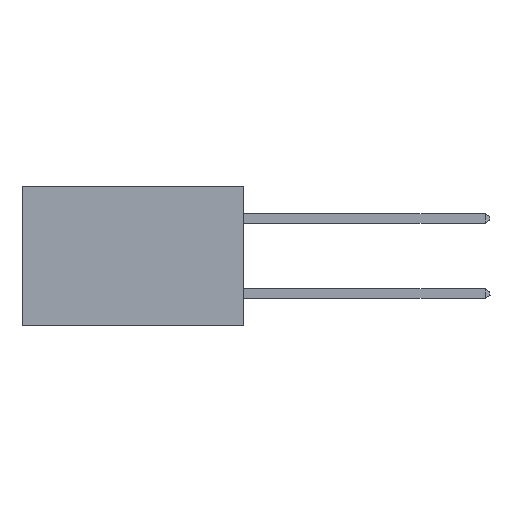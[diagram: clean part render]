
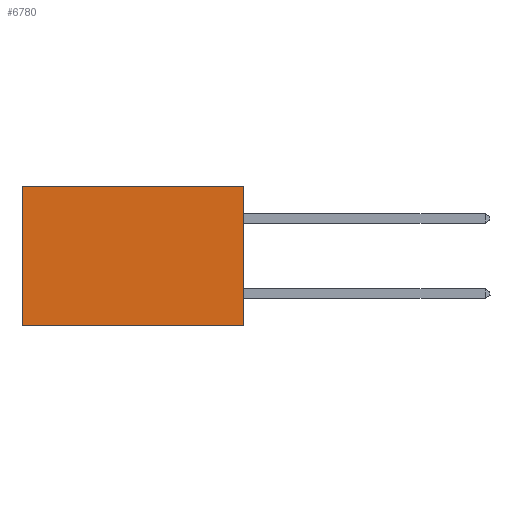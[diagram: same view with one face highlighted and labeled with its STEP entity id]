
A CAD part, left-side view. The second image highlights one B-rep face of the part: STEP entity #6780.
In plain terms, the highlighted planar face has unit normal (-1, 0, 0).
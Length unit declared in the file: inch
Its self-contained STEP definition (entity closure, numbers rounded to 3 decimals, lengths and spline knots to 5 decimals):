
#220 = AXIS2_PLACEMENT_3D ( 'NONE', #2139, #3180, #7868 ) ;
#2125 = CARTESIAN_POINT ( 'NONE',  ( 0.277, 0.59, -0.37 ) ) ;
#2139 = CARTESIAN_POINT ( 'NONE',  ( 0.277, 0., -0.37 ) ) ;
#2265 = FACE_OUTER_BOUND ( 'NONE', #10763, .T. ) ;
#2348 = LINE ( 'NONE', #7175, #12585 ) ;
#2513 = DIRECTION ( 'NONE',  ( 0., 0., -1. ) ) ;
#3180 = DIRECTION ( 'NONE',  ( 1., 0., 0. ) ) ;
#3348 = DIRECTION ( 'NONE',  ( 0., 1., 0. ) ) ;
#4469 = PLANE ( 'NONE',  #220 ) ;
#5017 = VERTEX_POINT ( 'NONE', #2125 ) ;
#6780 = ADVANCED_FACE ( 'NONE', ( #2265 ), #4469, .F. ) ;
#7138 = CARTESIAN_POINT ( 'NONE',  ( 0.277, 0., -0.37 ) ) ;
#7175 = CARTESIAN_POINT ( 'NONE',  ( 0.277, 0., 0. ) ) ;
#7466 = CARTESIAN_POINT ( 'NONE',  ( 0.277, 0., -0.37 ) ) ;
#7868 = DIRECTION ( 'NONE',  ( 0., 0., -1. ) ) ;
#7983 = LINE ( 'NONE', #7466, #13386 ) ;
#9213 = DIRECTION ( 'NONE',  ( 0., 1., 0. ) ) ;
#9620 = VECTOR ( 'NONE', #17366, 39.37008 ) ;
#10227 = EDGE_CURVE ( 'NONE', #17660, #12977, #2348, .T. ) ;
#10248 = LINE ( 'NONE', #7138, #9620 ) ;
#10322 = CARTESIAN_POINT ( 'NONE',  ( 0.277, 0.59, 0. ) ) ;
#10763 = EDGE_LOOP ( 'NONE', ( #21780, #11662, #16138, #25612 ) ) ;
#11537 = EDGE_CURVE ( 'NONE', #12977, #5017, #25639, .T. ) ;
#11662 = ORIENTED_EDGE ( 'NONE', *, *, #24642, .F. ) ;
#12585 = VECTOR ( 'NONE', #9213, 39.37008 ) ;
#12977 = VERTEX_POINT ( 'NONE', #10322 ) ;
#13386 = VECTOR ( 'NONE', #3348, 39.37008 ) ;
#16138 = ORIENTED_EDGE ( 'NONE', *, *, #18509, .F. ) ;
#17366 = DIRECTION ( 'NONE',  ( 0., 0., -1. ) ) ;
#17660 = VERTEX_POINT ( 'NONE', #18869 ) ;
#18509 = EDGE_CURVE ( 'NONE', #17660, #19380, #10248, .T. ) ;
#18869 = CARTESIAN_POINT ( 'NONE',  ( 0.277, 0., 0. ) ) ;
#18907 = CARTESIAN_POINT ( 'NONE',  ( 0.277, 0.59, -0.37 ) ) ;
#19380 = VERTEX_POINT ( 'NONE', #24280 ) ;
#19782 = VECTOR ( 'NONE', #2513, 39.37008 ) ;
#21780 = ORIENTED_EDGE ( 'NONE', *, *, #11537, .T. ) ;
#24280 = CARTESIAN_POINT ( 'NONE',  ( 0.277, 0., -0.37 ) ) ;
#24642 = EDGE_CURVE ( 'NONE', #19380, #5017, #7983, .T. ) ;
#25612 = ORIENTED_EDGE ( 'NONE', *, *, #10227, .T. ) ;
#25639 = LINE ( 'NONE', #18907, #19782 ) ;
